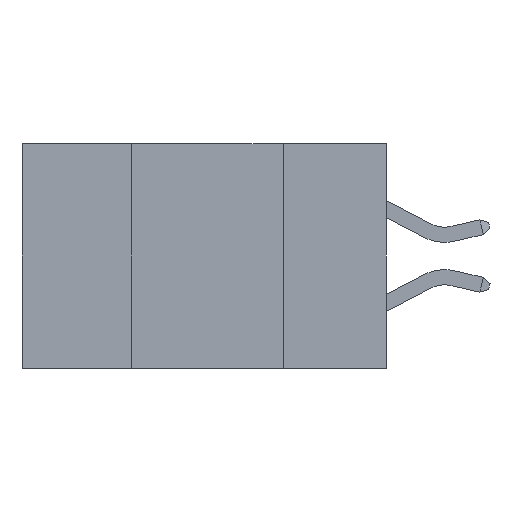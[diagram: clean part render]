
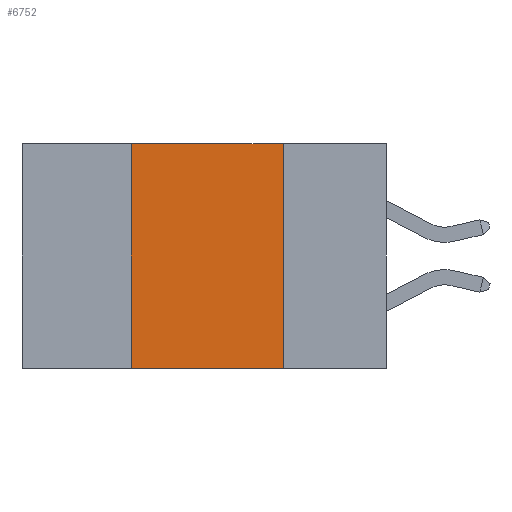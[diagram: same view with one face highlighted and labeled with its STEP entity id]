
A CAD part, left-side view. The second image highlights one B-rep face of the part: STEP entity #6752.
In plain terms, the highlighted planar face has unit normal (-1, 0, 0).
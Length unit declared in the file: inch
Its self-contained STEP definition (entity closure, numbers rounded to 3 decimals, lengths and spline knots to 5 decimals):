
#85 = CARTESIAN_POINT ( 'NONE',  ( 0., 0.42, 0. ) ) ;
#496 = CARTESIAN_POINT ( 'NONE',  ( 0., 0.6, -0.37 ) ) ;
#1348 = VECTOR ( 'NONE', #2669, 39.37008 ) ;
#1727 = DIRECTION ( 'NONE',  ( 0., 0., -1. ) ) ;
#2230 = ORIENTED_EDGE ( 'NONE', *, *, #5365, .F. ) ;
#2265 = VERTEX_POINT ( 'NONE', #5313 ) ;
#2331 = VECTOR ( 'NONE', #6852, 39.37008 ) ;
#2669 = DIRECTION ( 'NONE',  ( 0., -1., 0. ) ) ;
#2975 = CARTESIAN_POINT ( 'NONE',  ( 0., 0.17, 0. ) ) ;
#3692 = CARTESIAN_POINT ( 'NONE',  ( 0., 0.42, -0.37 ) ) ;
#3913 = ORIENTED_EDGE ( 'NONE', *, *, #8449, .T. ) ;
#4233 = LINE ( 'NONE', #496, #1348 ) ;
#4444 = PLANE ( 'NONE',  #12752 ) ;
#4470 = DIRECTION ( 'NONE',  ( 0., 0., 1. ) ) ;
#4483 = CARTESIAN_POINT ( 'NONE',  ( 0., 0.42, 0. ) ) ;
#5158 = FACE_OUTER_BOUND ( 'NONE', #12718, .T. ) ;
#5193 = LINE ( 'NONE', #2975, #10473 ) ;
#5198 = LINE ( 'NONE', #9061, #2331 ) ;
#5313 = CARTESIAN_POINT ( 'NONE',  ( 0., 0.17, 0. ) ) ;
#5365 = EDGE_CURVE ( 'NONE', #7316, #2265, #5198, .T. ) ;
#6162 = VERTEX_POINT ( 'NONE', #3692 ) ;
#6752 = ADVANCED_FACE ( 'NONE', ( #5158 ), #4444, .F. ) ;
#6852 = DIRECTION ( 'NONE',  ( 0., -1., 0. ) ) ;
#7316 = VERTEX_POINT ( 'NONE', #4483 ) ;
#7738 = DIRECTION ( 'NONE',  ( 1., 0., 0. ) ) ;
#7833 = VERTEX_POINT ( 'NONE', #10032 ) ;
#7913 = VECTOR ( 'NONE', #4470, 39.37008 ) ;
#8449 = EDGE_CURVE ( 'NONE', #6162, #7833, #4233, .T. ) ;
#8956 = CARTESIAN_POINT ( 'NONE',  ( 0., 0.6, 0. ) ) ;
#9061 = CARTESIAN_POINT ( 'NONE',  ( 0., 0.6, 0. ) ) ;
#9967 = DIRECTION ( 'NONE',  ( 0., 0., -1. ) ) ;
#10032 = CARTESIAN_POINT ( 'NONE',  ( 0., 0.17, -0.37 ) ) ;
#10332 = ORIENTED_EDGE ( 'NONE', *, *, #11585, .F. ) ;
#10473 = VECTOR ( 'NONE', #1727, 39.37008 ) ;
#10495 = EDGE_CURVE ( 'NONE', #2265, #7833, #5193, .T. ) ;
#10532 = ORIENTED_EDGE ( 'NONE', *, *, #10495, .F. ) ;
#10602 = LINE ( 'NONE', #85, #7913 ) ;
#11585 = EDGE_CURVE ( 'NONE', #6162, #7316, #10602, .T. ) ;
#12718 = EDGE_LOOP ( 'NONE', ( #10532, #2230, #10332, #3913 ) ) ;
#12752 = AXIS2_PLACEMENT_3D ( 'NONE', #8956, #7738, #9967 ) ;
